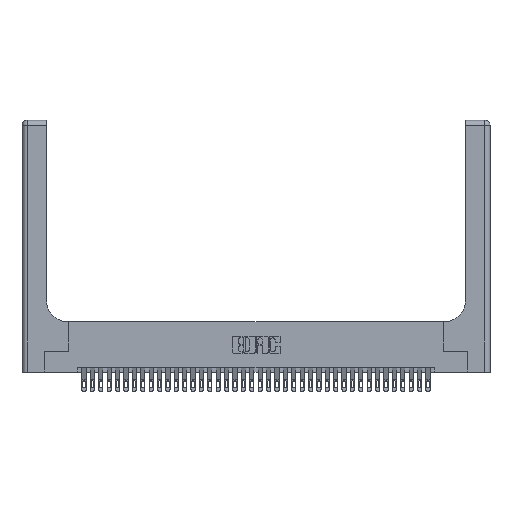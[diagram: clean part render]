
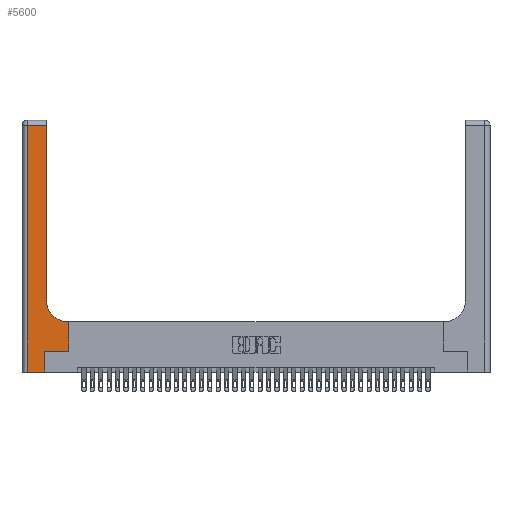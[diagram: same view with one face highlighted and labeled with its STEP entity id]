
A CAD part, top view. The second image highlights one B-rep face of the part: STEP entity #5600.
In plain terms, the highlighted planar face has unit normal (0, 0, 1).
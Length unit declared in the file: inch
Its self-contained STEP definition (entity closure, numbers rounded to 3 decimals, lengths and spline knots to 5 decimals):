
#13 = VERTEX_POINT ( 'NONE', #25124 ) ;
#397 = DIRECTION ( 'NONE',  ( 0., -1., 0. ) ) ;
#706 = ORIENTED_EDGE ( 'NONE', *, *, #3104, .T. ) ;
#825 = VERTEX_POINT ( 'NONE', #22714 ) ;
#1249 = AXIS2_PLACEMENT_3D ( 'NONE', #34846, #17564, #23175 ) ;
#3019 = VERTEX_POINT ( 'NONE', #16418 ) ;
#3104 = EDGE_CURVE ( 'NONE', #825, #38278, #21163, .T. ) ;
#3220 = EDGE_CURVE ( 'NONE', #3019, #13300, #12817, .T. ) ;
#3235 = VERTEX_POINT ( 'NONE', #33853 ) ;
#4140 = VECTOR ( 'NONE', #34183, 39.37008 ) ;
#4245 = ORIENTED_EDGE ( 'NONE', *, *, #29386, .T. ) ;
#4845 = PLANE ( 'NONE',  #19387 ) ;
#4865 = CARTESIAN_POINT ( 'NONE',  ( 0.5415, 0.6, 0.37 ) ) ;
#5594 = DIRECTION ( 'NONE',  ( 1., 0., 0. ) ) ;
#5600 = ADVANCED_FACE ( 'NONE', ( #19242 ), #4845, .F. ) ;
#5851 = LINE ( 'NONE', #30493, #36913 ) ;
#5894 = VECTOR ( 'NONE', #19926, 39.37008 ) ;
#6968 = VERTEX_POINT ( 'NONE', #14330 ) ;
#7511 = CIRCLE ( 'NONE', #1249, 0.25 ) ;
#7704 = DIRECTION ( 'NONE',  ( 0., 1., 0. ) ) ;
#7834 = VECTOR ( 'NONE', #28385, 39.37008 ) ;
#8898 = ORIENTED_EDGE ( 'NONE', *, *, #17609, .T. ) ;
#10161 = LINE ( 'NONE', #24496, #4140 ) ;
#10707 = ORIENTED_EDGE ( 'NONE', *, *, #21586, .T. ) ;
#12358 = VECTOR ( 'NONE', #7704, 39.37008 ) ;
#12495 = EDGE_CURVE ( 'NONE', #38278, #13, #37984, .T. ) ;
#12817 = LINE ( 'NONE', #25796, #5894 ) ;
#13300 = VERTEX_POINT ( 'NONE', #25141 ) ;
#13814 = DIRECTION ( 'NONE',  ( -1., 0., 0. ) ) ;
#14330 = CARTESIAN_POINT ( 'NONE',  ( 0.5585, 0.6, 0.37 ) ) ;
#15103 = EDGE_CURVE ( 'NONE', #3235, #3019, #22452, .T. ) ;
#16418 = CARTESIAN_POINT ( 'NONE',  ( 0.2915, 2.94, 0.37 ) ) ;
#17240 = EDGE_CURVE ( 'NONE', #13300, #29656, #28280, .T. ) ;
#17314 = ORIENTED_EDGE ( 'NONE', *, *, #15103, .T. ) ;
#17564 = DIRECTION ( 'NONE',  ( 0., 0., -1. ) ) ;
#17609 = EDGE_CURVE ( 'NONE', #6968, #36467, #30094, .T. ) ;
#17802 = VECTOR ( 'NONE', #26138, 39.37008 ) ;
#19242 = FACE_OUTER_BOUND ( 'NONE', #22167, .T. ) ;
#19387 = AXIS2_PLACEMENT_3D ( 'NONE', #31150, #19756, #13814 ) ;
#19463 = CARTESIAN_POINT ( 'NONE',  ( 0.269, 0., 0.37 ) ) ;
#19756 = DIRECTION ( 'NONE',  ( 0., 0., -1. ) ) ;
#19926 = DIRECTION ( 'NONE',  ( -1., 0., 0. ) ) ;
#21163 = LINE ( 'NONE', #19463, #12358 ) ;
#21586 = EDGE_CURVE ( 'NONE', #36467, #3235, #7511, .T. ) ;
#22167 = EDGE_LOOP ( 'NONE', ( #17314, #30903, #22827, #22907, #706, #26513, #4245, #8898, #10707 ) ) ;
#22452 = LINE ( 'NONE', #23394, #17802 ) ;
#22714 = CARTESIAN_POINT ( 'NONE',  ( 0.269, 0., 0.37 ) ) ;
#22827 = ORIENTED_EDGE ( 'NONE', *, *, #17240, .T. ) ;
#22907 = ORIENTED_EDGE ( 'NONE', *, *, #23651, .T. ) ;
#23175 = DIRECTION ( 'NONE',  ( 1., 0., 0. ) ) ;
#23394 = CARTESIAN_POINT ( 'NONE',  ( 0.2915, 3., 0.37 ) ) ;
#23651 = EDGE_CURVE ( 'NONE', #29656, #825, #10161, .T. ) ;
#24087 = CARTESIAN_POINT ( 'NONE',  ( 0.06, 3., 0.37 ) ) ;
#24139 = CARTESIAN_POINT ( 'NONE',  ( 0.269, 0.25, 0.37 ) ) ;
#24496 = CARTESIAN_POINT ( 'NONE',  ( 0., 0., 0.37 ) ) ;
#25124 = CARTESIAN_POINT ( 'NONE',  ( 0.5585, 0.25, 0.37 ) ) ;
#25141 = CARTESIAN_POINT ( 'NONE',  ( 0.06, 2.94, 0.37 ) ) ;
#25420 = CARTESIAN_POINT ( 'NONE',  ( 0.2915, 0.6, 0.37 ) ) ;
#25796 = CARTESIAN_POINT ( 'NONE',  ( 0., 2.94, 0.37 ) ) ;
#26128 = CARTESIAN_POINT ( 'NONE',  ( 0.06, 0., 0.37 ) ) ;
#26138 = DIRECTION ( 'NONE',  ( 0., 1., 0. ) ) ;
#26513 = ORIENTED_EDGE ( 'NONE', *, *, #12495, .T. ) ;
#28280 = LINE ( 'NONE', #24087, #36619 ) ;
#28385 = DIRECTION ( 'NONE',  ( -1., 0., 0. ) ) ;
#29386 = EDGE_CURVE ( 'NONE', #13, #6968, #5851, .T. ) ;
#29656 = VERTEX_POINT ( 'NONE', #26128 ) ;
#30038 = VECTOR ( 'NONE', #5594, 39.37008 ) ;
#30094 = LINE ( 'NONE', #25420, #7834 ) ;
#30493 = CARTESIAN_POINT ( 'NONE',  ( 0.5585, 0.25, 0.37 ) ) ;
#30736 = DIRECTION ( 'NONE',  ( 0., 1., 0. ) ) ;
#30903 = ORIENTED_EDGE ( 'NONE', *, *, #3220, .T. ) ;
#31150 = CARTESIAN_POINT ( 'NONE',  ( 0., 3., 0.37 ) ) ;
#33853 = CARTESIAN_POINT ( 'NONE',  ( 0.2915, 0.85, 0.37 ) ) ;
#34183 = DIRECTION ( 'NONE',  ( 1., 0., 0. ) ) ;
#34846 = CARTESIAN_POINT ( 'NONE',  ( 0.5415, 0.85, 0.37 ) ) ;
#36467 = VERTEX_POINT ( 'NONE', #4865 ) ;
#36619 = VECTOR ( 'NONE', #397, 39.37008 ) ;
#36913 = VECTOR ( 'NONE', #30736, 39.37008 ) ;
#37984 = LINE ( 'NONE', #38047, #30038 ) ;
#38047 = CARTESIAN_POINT ( 'NONE',  ( 0.269, 0.25, 0.37 ) ) ;
#38278 = VERTEX_POINT ( 'NONE', #24139 ) ;
